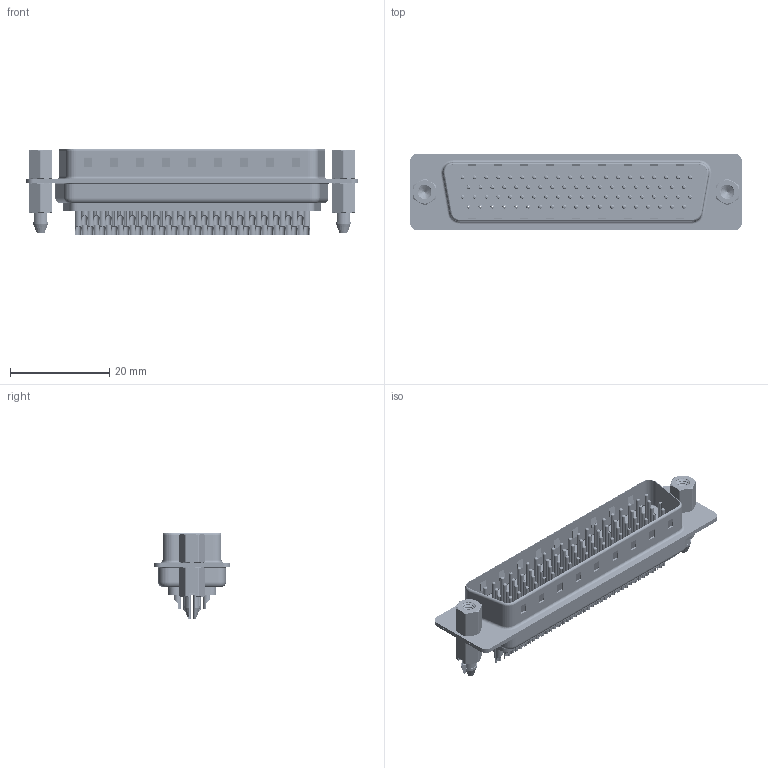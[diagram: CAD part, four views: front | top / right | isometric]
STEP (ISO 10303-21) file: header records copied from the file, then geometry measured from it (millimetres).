
FILE_DESCRIPTION (( 'STEP AP203' ), '1' );
FILE_NAME ('637-078-632-247.STEP', '2020-07-18T06:42:32', ( '' ), ( '' ), 'SwSTEP 2.0', 'SolidWorks 2020', '' );
FILE_SCHEMA (( 'CONFIG_CONTROL_DESIGN' ));
Length unit declared in the file: millimetre
Products named in the file (10): 637 Contact Row 78_32; 637-078-632-247; 637 Shell Rear_78 Contacts; 637 Contact Row 3_32; 637 Contact Row 2_32(78); 637 Housing_78 Contacts; 637 Shell Front_78 Contacts; 637 4-40 Threaded Boardlock_LP; 637 4-40 Hex Standoff; 637 Contact Row 1_32(78)
Assembly tree (85 placements, depth 2):
  637-078-632-247
    637 Housing_78 Contacts
    637 Shell Front_78 Contacts
    637 Shell Rear_78 Contacts
    637 Contact Row 1_32(78)  x19
    637 Contact Row 2_32(78)  x20
    637 Contact Row 3_32  x19
    637 Contact Row 78_32  x20
    637 4-40 Hex Standoff  x2
    637 4-40 Threaded Boardlock_LP  x2
Bounding box: 67 x 15.4 x 17.55 mm (x, y, z)
Volume: 4759.3 mm3; surface area: 17547.9 mm2
Topology: 85 solids, 85 shells, 5604 faces, 14429 edges, 9160 vertices
Faces by surface type: cylinder 2507, torus 1688, plane 1349, cone 42, bspline 18
Entity records: 47399 total; most frequent: CARTESIAN_POINT 11271, DIRECTION 7456, ORIENTED_EDGE 6504, EDGE_CURVE 3252, AXIS2_PLACEMENT_3D 3027, VERTEX_POINT 2109, EDGE_LOOP 1699, CIRCLE 1621
